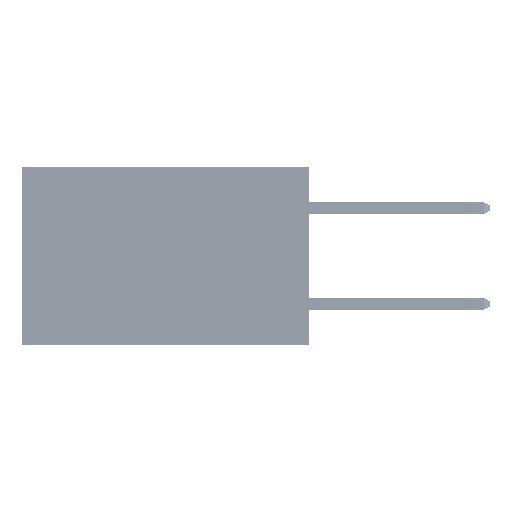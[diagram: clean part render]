
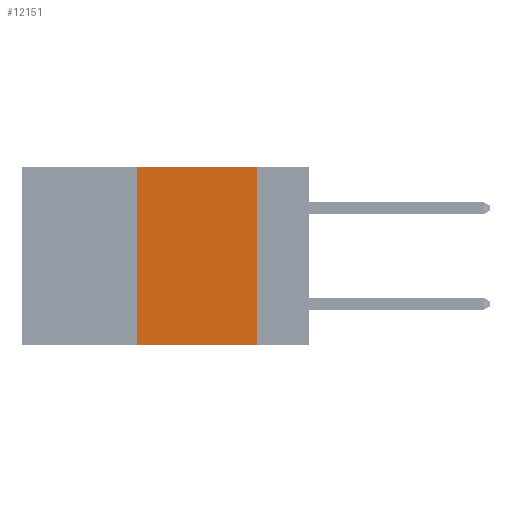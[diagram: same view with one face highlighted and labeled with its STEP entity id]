
A CAD part, left-side view. The second image highlights one B-rep face of the part: STEP entity #12151.
In plain terms, the highlighted planar face has unit normal (-1, 0, 0).
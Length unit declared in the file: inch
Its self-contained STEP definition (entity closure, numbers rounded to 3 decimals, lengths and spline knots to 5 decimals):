
#933 = LINE ( 'NONE', #21667, #37142 ) ;
#1340 = VECTOR ( 'NONE', #6904, 39.37008 ) ;
#1985 = ORIENTED_EDGE ( 'NONE', *, *, #38092, .F. ) ;
#3101 = CARTESIAN_POINT ( 'NONE',  ( 0., 0.6, -0.37 ) ) ;
#4887 = LINE ( 'NONE', #3101, #1340 ) ;
#5387 = CARTESIAN_POINT ( 'NONE',  ( 0., 0.36, 0. ) ) ;
#6766 = CARTESIAN_POINT ( 'NONE',  ( 0., 0.36, 0. ) ) ;
#6904 = DIRECTION ( 'NONE',  ( 0., -1., 0. ) ) ;
#7138 = PLANE ( 'NONE',  #40470 ) ;
#7251 = VERTEX_POINT ( 'NONE', #39670 ) ;
#10390 = EDGE_CURVE ( 'NONE', #47370, #46222, #933, .T. ) ;
#10566 = DIRECTION ( 'NONE',  ( 0., 0., 1. ) ) ;
#10920 = CARTESIAN_POINT ( 'NONE',  ( 0., 0.6, 0. ) ) ;
#12151 = ADVANCED_FACE ( 'NONE', ( #30096 ), #7138, .F. ) ;
#13464 = VECTOR ( 'NONE', #10566, 39.37008 ) ;
#14681 = DIRECTION ( 'NONE',  ( 0., 0., -1. ) ) ;
#15354 = ORIENTED_EDGE ( 'NONE', *, *, #19953, .F. ) ;
#17155 = VECTOR ( 'NONE', #25672, 39.37008 ) ;
#17648 = CARTESIAN_POINT ( 'NONE',  ( 0., 0.11, 0. ) ) ;
#19360 = EDGE_LOOP ( 'NONE', ( #1985, #29123, #15354, #32499 ) ) ;
#19953 = EDGE_CURVE ( 'NONE', #47603, #47370, #43068, .T. ) ;
#21667 = CARTESIAN_POINT ( 'NONE',  ( 0., 0.6, 0. ) ) ;
#25416 = DIRECTION ( 'NONE',  ( 0., -1., 0. ) ) ;
#25505 = CARTESIAN_POINT ( 'NONE',  ( 0., 0.36, -0.37 ) ) ;
#25672 = DIRECTION ( 'NONE',  ( 0., 0., -1. ) ) ;
#29123 = ORIENTED_EDGE ( 'NONE', *, *, #10390, .F. ) ;
#30096 = FACE_OUTER_BOUND ( 'NONE', #19360, .T. ) ;
#32499 = ORIENTED_EDGE ( 'NONE', *, *, #37346, .T. ) ;
#36892 = LINE ( 'NONE', #47674, #17155 ) ;
#36958 = DIRECTION ( 'NONE',  ( 1., 0., 0. ) ) ;
#37142 = VECTOR ( 'NONE', #25416, 39.37008 ) ;
#37346 = EDGE_CURVE ( 'NONE', #47603, #7251, #4887, .T. ) ;
#38092 = EDGE_CURVE ( 'NONE', #46222, #7251, #36892, .T. ) ;
#39670 = CARTESIAN_POINT ( 'NONE',  ( 0., 0.11, -0.37 ) ) ;
#40470 = AXIS2_PLACEMENT_3D ( 'NONE', #10920, #36958, #14681 ) ;
#43068 = LINE ( 'NONE', #6766, #13464 ) ;
#46222 = VERTEX_POINT ( 'NONE', #17648 ) ;
#47370 = VERTEX_POINT ( 'NONE', #5387 ) ;
#47603 = VERTEX_POINT ( 'NONE', #25505 ) ;
#47674 = CARTESIAN_POINT ( 'NONE',  ( 0., 0.11, 0. ) ) ;
